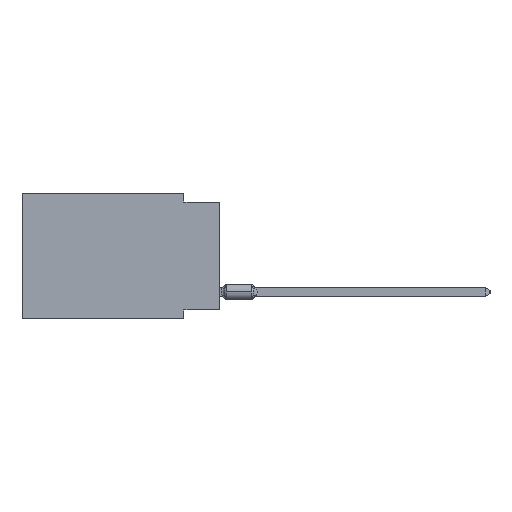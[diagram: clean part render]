
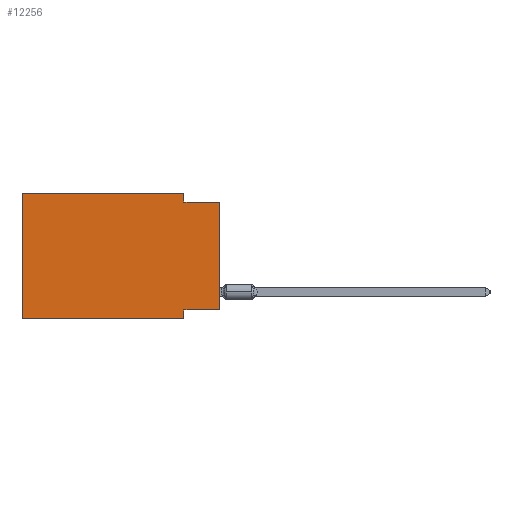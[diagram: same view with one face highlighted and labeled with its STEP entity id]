
A CAD part, left-side view. The second image highlights one B-rep face of the part: STEP entity #12256.
In plain terms, the highlighted planar face has unit normal (-1, 0, 0).
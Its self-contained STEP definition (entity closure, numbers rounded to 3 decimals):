
#1954 = DIRECTION ( 'NONE',  ( 0., 0., -1. ) ) ;
#2368 = DIRECTION ( 'NONE',  ( 1., 0., 0. ) ) ;
#3067 = DIRECTION ( 'NONE',  ( 0., -1., 0. ) ) ;
#5099 = CARTESIAN_POINT ( 'NONE',  ( 0., 2.54, -0.635 ) ) ;
#5641 = EDGE_CURVE ( 'NONE', #40538, #45700, #82505, .T. ) ;
#6845 = VECTOR ( 'NONE', #83874, 1000. ) ;
#8733 = ORIENTED_EDGE ( 'NONE', *, *, #28325, .F. ) ;
#9267 = CARTESIAN_POINT ( 'NONE',  ( 0., 13.97, 0. ) ) ;
#10644 = ORIENTED_EDGE ( 'NONE', *, *, #64316, .F. ) ;
#11407 = EDGE_CURVE ( 'NONE', #78800, #69354, #45988, .T. ) ;
#12256 = ADVANCED_FACE ( 'NONE', ( #41093 ), #54556, .F. ) ;
#13194 = LINE ( 'NONE', #20142, #14968 ) ;
#13372 = CARTESIAN_POINT ( 'NONE',  ( 0., 0., -8.255 ) ) ;
#14968 = VECTOR ( 'NONE', #46659, 1000. ) ;
#16849 = CARTESIAN_POINT ( 'NONE',  ( 0., 13.97, 0. ) ) ;
#16954 = ORIENTED_EDGE ( 'NONE', *, *, #59229, .T. ) ;
#18053 = ORIENTED_EDGE ( 'NONE', *, *, #51297, .T. ) ;
#19999 = EDGE_CURVE ( 'NONE', #45700, #35052, #25253, .T. ) ;
#20142 = CARTESIAN_POINT ( 'NONE',  ( 0., 0., 0. ) ) ;
#22108 = LINE ( 'NONE', #35987, #65520 ) ;
#22144 = DIRECTION ( 'NONE',  ( 0., 0., 1. ) ) ;
#22161 = CARTESIAN_POINT ( 'NONE',  ( 0., 2.54, -8.255 ) ) ;
#25253 = LINE ( 'NONE', #43967, #76322 ) ;
#25715 = VECTOR ( 'NONE', #69030, 1000. ) ;
#25922 = ORIENTED_EDGE ( 'NONE', *, *, #19999, .F. ) ;
#26170 = CARTESIAN_POINT ( 'NONE',  ( 0., 13.97, 0. ) ) ;
#26442 = VERTEX_POINT ( 'NONE', #65827 ) ;
#27640 = ORIENTED_EDGE ( 'NONE', *, *, #11407, .F. ) ;
#28325 = EDGE_CURVE ( 'NONE', #35052, #75987, #36984, .T. ) ;
#29458 = VECTOR ( 'NONE', #22144, 1000. ) ;
#30474 = AXIS2_PLACEMENT_3D ( 'NONE', #53260, #2368, #1954 ) ;
#35046 = EDGE_LOOP ( 'NONE', ( #16954, #8733, #25922, #39097, #50146, #18053, #10644, #27640 ) ) ;
#35052 = VERTEX_POINT ( 'NONE', #5099 ) ;
#35987 = CARTESIAN_POINT ( 'NONE',  ( 0., 13.97, -8.89 ) ) ;
#36984 = LINE ( 'NONE', #62624, #84215 ) ;
#39097 = ORIENTED_EDGE ( 'NONE', *, *, #5641, .F. ) ;
#40538 = VERTEX_POINT ( 'NONE', #9267 ) ;
#40638 = CARTESIAN_POINT ( 'NONE',  ( 0., 0., -0.635 ) ) ;
#41093 = FACE_OUTER_BOUND ( 'NONE', #35046, .T. ) ;
#42521 = DIRECTION ( 'NONE',  ( 0., -1., 0. ) ) ;
#42826 = EDGE_CURVE ( 'NONE', #26442, #40538, #75168, .T. ) ;
#43967 = CARTESIAN_POINT ( 'NONE',  ( 0., 2.54, 0. ) ) ;
#45700 = VERTEX_POINT ( 'NONE', #52664 ) ;
#45988 = LINE ( 'NONE', #13372, #78957 ) ;
#46659 = DIRECTION ( 'NONE',  ( 0., 0., 1. ) ) ;
#50146 = ORIENTED_EDGE ( 'NONE', *, *, #42826, .F. ) ;
#51297 = EDGE_CURVE ( 'NONE', #26442, #82463, #22108, .T. ) ;
#52664 = CARTESIAN_POINT ( 'NONE',  ( 0., 2.54, 0. ) ) ;
#53260 = CARTESIAN_POINT ( 'NONE',  ( 0., 13.97, 0. ) ) ;
#54556 = PLANE ( 'NONE',  #30474 ) ;
#59052 = CARTESIAN_POINT ( 'NONE',  ( 0., 2.54, -8.89 ) ) ;
#59229 = EDGE_CURVE ( 'NONE', #78800, #75987, #13194, .T. ) ;
#62624 = CARTESIAN_POINT ( 'NONE',  ( 0., 0., -0.635 ) ) ;
#64316 = EDGE_CURVE ( 'NONE', #69354, #82463, #82586, .T. ) ;
#65520 = VECTOR ( 'NONE', #42521, 1000. ) ;
#65827 = CARTESIAN_POINT ( 'NONE',  ( 0., 13.97, -8.89 ) ) ;
#69030 = DIRECTION ( 'NONE',  ( 0., -1., 0. ) ) ;
#69354 = VERTEX_POINT ( 'NONE', #22161 ) ;
#70391 = CARTESIAN_POINT ( 'NONE',  ( 0., 2.54, -8.89 ) ) ;
#72928 = DIRECTION ( 'NONE',  ( 0., 1., 0. ) ) ;
#73646 = CARTESIAN_POINT ( 'NONE',  ( 0., 0., -8.255 ) ) ;
#75168 = LINE ( 'NONE', #26170, #29458 ) ;
#75987 = VERTEX_POINT ( 'NONE', #40638 ) ;
#76322 = VECTOR ( 'NONE', #84816, 1000. ) ;
#78800 = VERTEX_POINT ( 'NONE', #73646 ) ;
#78957 = VECTOR ( 'NONE', #72928, 1000. ) ;
#82463 = VERTEX_POINT ( 'NONE', #59052 ) ;
#82505 = LINE ( 'NONE', #16849, #25715 ) ;
#82586 = LINE ( 'NONE', #70391, #6845 ) ;
#83874 = DIRECTION ( 'NONE',  ( 0., 0., -1. ) ) ;
#84215 = VECTOR ( 'NONE', #3067, 1000. ) ;
#84816 = DIRECTION ( 'NONE',  ( 0., 0., -1. ) ) ;
